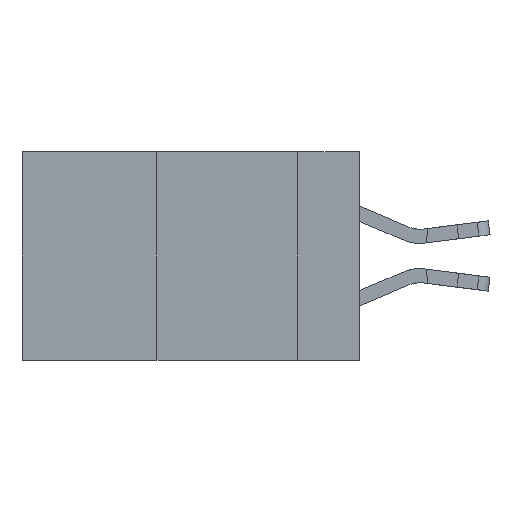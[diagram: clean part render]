
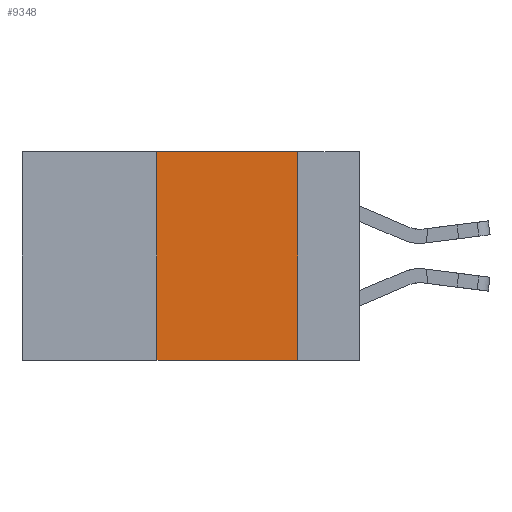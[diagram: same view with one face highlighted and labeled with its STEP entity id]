
A CAD part, left-side view. The second image highlights one B-rep face of the part: STEP entity #9348.
In plain terms, the highlighted planar face has unit normal (-1, 0, 0).
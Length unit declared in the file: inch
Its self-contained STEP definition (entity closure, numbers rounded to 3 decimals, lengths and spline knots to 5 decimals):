
#349 = DIRECTION ( 'NONE',  ( 0., -1., 0. ) ) ;
#776 = VECTOR ( 'NONE', #349, 39.37008 ) ;
#809 = CARTESIAN_POINT ( 'NONE',  ( 0., 0.6, -0.37 ) ) ;
#1498 = DIRECTION ( 'NONE',  ( 0., -1., 0. ) ) ;
#1682 = LINE ( 'NONE', #16597, #776 ) ;
#2256 = LINE ( 'NONE', #21967, #6348 ) ;
#2384 = LINE ( 'NONE', #7825, #14550 ) ;
#4491 = DIRECTION ( 'NONE',  ( 0., 0., -1. ) ) ;
#5094 = CARTESIAN_POINT ( 'NONE',  ( 0., 0.36, -0.37 ) ) ;
#5186 = ORIENTED_EDGE ( 'NONE', *, *, #14821, .F. ) ;
#5852 = CARTESIAN_POINT ( 'NONE',  ( 0., 0.36, 0. ) ) ;
#6348 = VECTOR ( 'NONE', #9512, 39.37008 ) ;
#7000 = ORIENTED_EDGE ( 'NONE', *, *, #22187, .T. ) ;
#7825 = CARTESIAN_POINT ( 'NONE',  ( 0., 0.11, 0. ) ) ;
#8805 = AXIS2_PLACEMENT_3D ( 'NONE', #9934, #11331, #17149 ) ;
#9035 = CARTESIAN_POINT ( 'NONE',  ( 0., 0.11, -0.37 ) ) ;
#9348 = ADVANCED_FACE ( 'NONE', ( #17015 ), #22730, .F. ) ;
#9512 = DIRECTION ( 'NONE',  ( 0., 0., 1. ) ) ;
#9920 = VERTEX_POINT ( 'NONE', #10437 ) ;
#9934 = CARTESIAN_POINT ( 'NONE',  ( 0., 0.6, 0. ) ) ;
#10437 = CARTESIAN_POINT ( 'NONE',  ( 0., 0.11, 0. ) ) ;
#11331 = DIRECTION ( 'NONE',  ( 1., 0., 0. ) ) ;
#11515 = EDGE_CURVE ( 'NONE', #18720, #9920, #1682, .T. ) ;
#12886 = ORIENTED_EDGE ( 'NONE', *, *, #11515, .F. ) ;
#13111 = ORIENTED_EDGE ( 'NONE', *, *, #15814, .F. ) ;
#14550 = VECTOR ( 'NONE', #4491, 39.37008 ) ;
#14821 = EDGE_CURVE ( 'NONE', #9920, #21375, #2384, .T. ) ;
#15487 = VECTOR ( 'NONE', #1498, 39.37008 ) ;
#15814 = EDGE_CURVE ( 'NONE', #17242, #18720, #2256, .T. ) ;
#16377 = EDGE_LOOP ( 'NONE', ( #5186, #12886, #13111, #7000 ) ) ;
#16597 = CARTESIAN_POINT ( 'NONE',  ( 0., 0.6, 0. ) ) ;
#17015 = FACE_OUTER_BOUND ( 'NONE', #16377, .T. ) ;
#17149 = DIRECTION ( 'NONE',  ( 0., 0., -1. ) ) ;
#17242 = VERTEX_POINT ( 'NONE', #5094 ) ;
#18720 = VERTEX_POINT ( 'NONE', #5852 ) ;
#20643 = LINE ( 'NONE', #809, #15487 ) ;
#21375 = VERTEX_POINT ( 'NONE', #9035 ) ;
#21967 = CARTESIAN_POINT ( 'NONE',  ( 0., 0.36, 0. ) ) ;
#22187 = EDGE_CURVE ( 'NONE', #17242, #21375, #20643, .T. ) ;
#22730 = PLANE ( 'NONE',  #8805 ) ;
